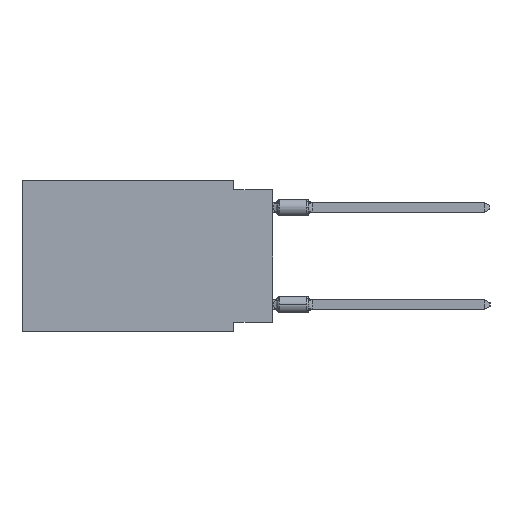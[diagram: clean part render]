
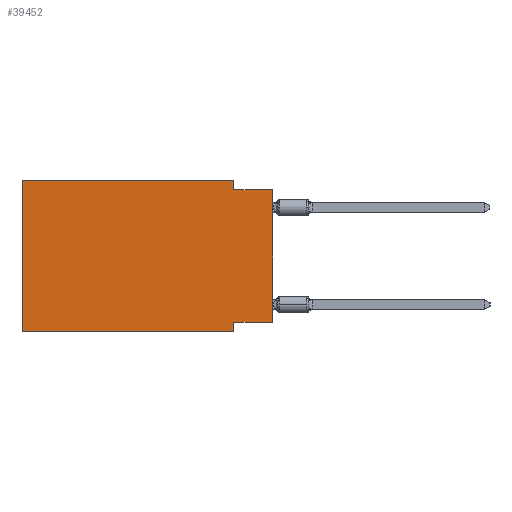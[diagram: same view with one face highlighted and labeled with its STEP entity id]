
A CAD part, left-side view. The second image highlights one B-rep face of the part: STEP entity #39452.
In plain terms, the highlighted planar face has unit normal (-1, 0, 0).
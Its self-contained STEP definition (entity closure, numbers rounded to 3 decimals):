
#308 = VECTOR ( 'NONE', #11870, 1000. ) ;
#1003 = VERTEX_POINT ( 'NONE', #31719 ) ;
#1238 = VERTEX_POINT ( 'NONE', #34105 ) ;
#1336 = PLANE ( 'NONE',  #7039 ) ;
#1831 = ORIENTED_EDGE ( 'NONE', *, *, #31249, .F. ) ;
#1882 = VECTOR ( 'NONE', #17907, 1000. ) ;
#2801 = VECTOR ( 'NONE', #28992, 1000. ) ;
#3505 = ORIENTED_EDGE ( 'NONE', *, *, #10957, .F. ) ;
#5347 = EDGE_CURVE ( 'NONE', #36674, #1003, #11955, .T. ) ;
#5533 = CARTESIAN_POINT ( 'NONE',  ( 0., 0., -9.271 ) ) ;
#5594 = LINE ( 'NONE', #24560, #1882 ) ;
#6125 = DIRECTION ( 'NONE',  ( 0., -1., 0. ) ) ;
#6744 = DIRECTION ( 'NONE',  ( 0., 0., -1. ) ) ;
#6891 = CARTESIAN_POINT ( 'NONE',  ( 0., 16.383, 0. ) ) ;
#7039 = AXIS2_PLACEMENT_3D ( 'NONE', #47157, #13433, #45780 ) ;
#7489 = EDGE_CURVE ( 'NONE', #1003, #41072, #14494, .T. ) ;
#9271 = DIRECTION ( 'NONE',  ( 0., 1., 0. ) ) ;
#10148 = VERTEX_POINT ( 'NONE', #16155 ) ;
#10390 = LINE ( 'NONE', #29309, #27821 ) ;
#10934 = VECTOR ( 'NONE', #33663, 1000. ) ;
#10957 = EDGE_CURVE ( 'NONE', #1238, #10148, #44273, .T. ) ;
#11870 = DIRECTION ( 'NONE',  ( 0., 0., 1. ) ) ;
#11955 = LINE ( 'NONE', #45915, #25091 ) ;
#12051 = CARTESIAN_POINT ( 'NONE',  ( 0., 16.383, -9.906 ) ) ;
#12085 = VERTEX_POINT ( 'NONE', #42201 ) ;
#13143 = ORIENTED_EDGE ( 'NONE', *, *, #28485, .T. ) ;
#13433 = DIRECTION ( 'NONE',  ( 1., 0., 0. ) ) ;
#13825 = EDGE_LOOP ( 'NONE', ( #13143, #39322, #1831, #3505, #38511, #16561, #23554, #27117 ) ) ;
#14494 = LINE ( 'NONE', #43893, #20589 ) ;
#16155 = CARTESIAN_POINT ( 'NONE',  ( 0., 2.54, 0. ) ) ;
#16561 = ORIENTED_EDGE ( 'NONE', *, *, #33955, .T. ) ;
#17907 = DIRECTION ( 'NONE',  ( 0., 0., 1. ) ) ;
#20548 = CARTESIAN_POINT ( 'NONE',  ( 0., 0., -0.635 ) ) ;
#20589 = VECTOR ( 'NONE', #22014, 1000. ) ;
#20885 = EDGE_CURVE ( 'NONE', #43668, #23736, #39392, .T. ) ;
#22014 = DIRECTION ( 'NONE',  ( 0., 0., -1. ) ) ;
#23554 = ORIENTED_EDGE ( 'NONE', *, *, #7489, .F. ) ;
#23736 = VERTEX_POINT ( 'NONE', #20548 ) ;
#24560 = CARTESIAN_POINT ( 'NONE',  ( 0., 16.383, 0. ) ) ;
#25091 = VECTOR ( 'NONE', #9271, 1000. ) ;
#25723 = CARTESIAN_POINT ( 'NONE',  ( 0., 0., 0. ) ) ;
#27117 = ORIENTED_EDGE ( 'NONE', *, *, #5347, .F. ) ;
#27533 = CARTESIAN_POINT ( 'NONE',  ( 0., 2.54, -9.906 ) ) ;
#27749 = CARTESIAN_POINT ( 'NONE',  ( 0., 0., -0.635 ) ) ;
#27821 = VECTOR ( 'NONE', #6744, 1000. ) ;
#28485 = EDGE_CURVE ( 'NONE', #36674, #23736, #44178, .T. ) ;
#28992 = DIRECTION ( 'NONE',  ( 0., -1., 0. ) ) ;
#29309 = CARTESIAN_POINT ( 'NONE',  ( 0., 2.54, 0. ) ) ;
#31249 = EDGE_CURVE ( 'NONE', #10148, #43668, #10390, .T. ) ;
#31719 = CARTESIAN_POINT ( 'NONE',  ( 0., 2.54, -9.271 ) ) ;
#31956 = VECTOR ( 'NONE', #6125, 1000. ) ;
#33445 = CARTESIAN_POINT ( 'NONE',  ( 0., 2.54, -0.635 ) ) ;
#33663 = DIRECTION ( 'NONE',  ( 0., -1., 0. ) ) ;
#33955 = EDGE_CURVE ( 'NONE', #12085, #41072, #37287, .T. ) ;
#34105 = CARTESIAN_POINT ( 'NONE',  ( 0., 16.383, 0. ) ) ;
#36674 = VERTEX_POINT ( 'NONE', #5533 ) ;
#37287 = LINE ( 'NONE', #12051, #10934 ) ;
#38511 = ORIENTED_EDGE ( 'NONE', *, *, #45840, .F. ) ;
#39322 = ORIENTED_EDGE ( 'NONE', *, *, #20885, .F. ) ;
#39392 = LINE ( 'NONE', #27749, #31956 ) ;
#39452 = ADVANCED_FACE ( 'NONE', ( #42158 ), #1336, .F. ) ;
#41072 = VERTEX_POINT ( 'NONE', #27533 ) ;
#42158 = FACE_OUTER_BOUND ( 'NONE', #13825, .T. ) ;
#42201 = CARTESIAN_POINT ( 'NONE',  ( 0., 16.383, -9.906 ) ) ;
#43668 = VERTEX_POINT ( 'NONE', #33445 ) ;
#43893 = CARTESIAN_POINT ( 'NONE',  ( 0., 2.54, -9.906 ) ) ;
#44178 = LINE ( 'NONE', #25723, #308 ) ;
#44273 = LINE ( 'NONE', #6891, #2801 ) ;
#45780 = DIRECTION ( 'NONE',  ( 0., 0., -1. ) ) ;
#45840 = EDGE_CURVE ( 'NONE', #12085, #1238, #5594, .T. ) ;
#45915 = CARTESIAN_POINT ( 'NONE',  ( 0., 0., -9.271 ) ) ;
#47157 = CARTESIAN_POINT ( 'NONE',  ( 0., 16.383, 0. ) ) ;
